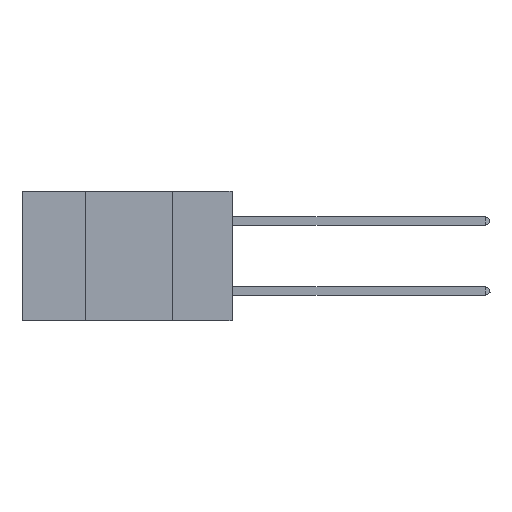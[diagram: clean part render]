
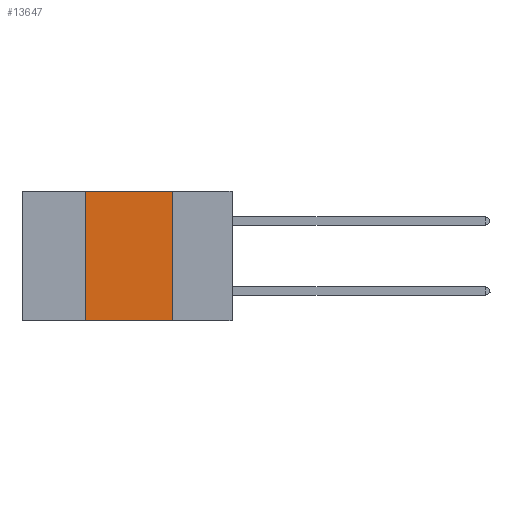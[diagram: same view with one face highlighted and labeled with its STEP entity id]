
A CAD part, left-side view. The second image highlights one B-rep face of the part: STEP entity #13647.
In plain terms, the highlighted planar face has unit normal (-1, 0, 0).
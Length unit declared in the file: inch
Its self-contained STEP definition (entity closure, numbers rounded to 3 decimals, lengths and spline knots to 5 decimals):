
#359 = PLANE ( 'NONE',  #2699 ) ;
#734 = CARTESIAN_POINT ( 'NONE',  ( 0., 0.17, 0. ) ) ;
#762 = DIRECTION ( 'NONE',  ( 0., 0., -1. ) ) ;
#1252 = VECTOR ( 'NONE', #8284, 39.37008 ) ;
#1450 = EDGE_CURVE ( 'NONE', #3439, #14219, #5775, .T. ) ;
#1468 = ORIENTED_EDGE ( 'NONE', *, *, #1450, .F. ) ;
#1548 = ORIENTED_EDGE ( 'NONE', *, *, #12628, .F. ) ;
#1599 = ORIENTED_EDGE ( 'NONE', *, *, #15278, .F. ) ;
#1641 = DIRECTION ( 'NONE',  ( 0., 0., -1. ) ) ;
#1654 = LINE ( 'NONE', #7067, #1252 ) ;
#1708 = ORIENTED_EDGE ( 'NONE', *, *, #14510, .T. ) ;
#2303 = VECTOR ( 'NONE', #13927, 39.37008 ) ;
#2699 = AXIS2_PLACEMENT_3D ( 'NONE', #11231, #8960, #1641 ) ;
#2954 = VECTOR ( 'NONE', #6896, 39.37008 ) ;
#3439 = VERTEX_POINT ( 'NONE', #6980 ) ;
#4350 = VERTEX_POINT ( 'NONE', #10902 ) ;
#5388 = VECTOR ( 'NONE', #762, 39.37008 ) ;
#5669 = CARTESIAN_POINT ( 'NONE',  ( 0., 0.6, -0.37 ) ) ;
#5775 = LINE ( 'NONE', #734, #5388 ) ;
#6896 = DIRECTION ( 'NONE',  ( 0., -1., 0. ) ) ;
#6980 = CARTESIAN_POINT ( 'NONE',  ( 0., 0.17, 0. ) ) ;
#7067 = CARTESIAN_POINT ( 'NONE',  ( 0., 0.42, 0. ) ) ;
#8284 = DIRECTION ( 'NONE',  ( 0., 0., 1. ) ) ;
#8960 = DIRECTION ( 'NONE',  ( 1., 0., 0. ) ) ;
#9211 = EDGE_LOOP ( 'NONE', ( #1468, #1548, #1599, #1708 ) ) ;
#9297 = CARTESIAN_POINT ( 'NONE',  ( 0., 0.6, 0. ) ) ;
#9376 = LINE ( 'NONE', #9297, #2954 ) ;
#10162 = CARTESIAN_POINT ( 'NONE',  ( 0., 0.42, 0. ) ) ;
#10902 = CARTESIAN_POINT ( 'NONE',  ( 0., 0.42, -0.37 ) ) ;
#11231 = CARTESIAN_POINT ( 'NONE',  ( 0., 0.6, 0. ) ) ;
#12222 = CARTESIAN_POINT ( 'NONE',  ( 0., 0.17, -0.37 ) ) ;
#12628 = EDGE_CURVE ( 'NONE', #13676, #3439, #9376, .T. ) ;
#12951 = FACE_OUTER_BOUND ( 'NONE', #9211, .T. ) ;
#13647 = ADVANCED_FACE ( 'NONE', ( #12951 ), #359, .F. ) ;
#13676 = VERTEX_POINT ( 'NONE', #10162 ) ;
#13927 = DIRECTION ( 'NONE',  ( 0., -1., 0. ) ) ;
#14219 = VERTEX_POINT ( 'NONE', #12222 ) ;
#14510 = EDGE_CURVE ( 'NONE', #4350, #14219, #14880, .T. ) ;
#14880 = LINE ( 'NONE', #5669, #2303 ) ;
#15278 = EDGE_CURVE ( 'NONE', #4350, #13676, #1654, .T. ) ;
